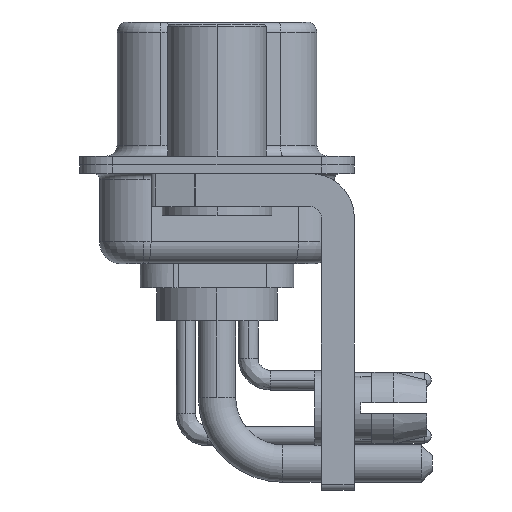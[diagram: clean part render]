
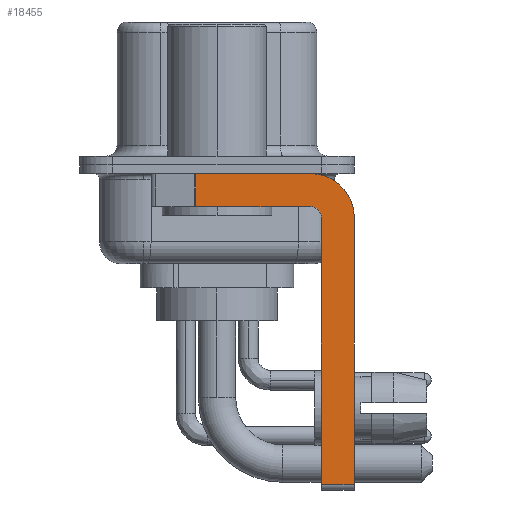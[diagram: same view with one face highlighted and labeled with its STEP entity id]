
A CAD part, left-side view. The second image highlights one B-rep face of the part: STEP entity #18455.
In plain terms, the highlighted planar face has unit normal (-1, 0, 0).
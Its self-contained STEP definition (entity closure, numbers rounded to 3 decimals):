
#10 = VECTOR ( 'NONE', #18727, 1000. ) ;
#968 = VERTEX_POINT ( 'NONE', #21415 ) ;
#1246 = LINE ( 'NONE', #16318, #1496 ) ;
#1315 = ORIENTED_EDGE ( 'NONE', *, *, #11298, .F. ) ;
#1330 = DIRECTION ( 'NONE',  ( 0., 0., -1. ) ) ;
#1350 = DIRECTION ( 'NONE',  ( 0., 0., -1. ) ) ;
#1496 = VECTOR ( 'NONE', #17808, 1000. ) ;
#1505 = LINE ( 'NONE', #12871, #17289 ) ;
#2481 = CARTESIAN_POINT ( 'NONE',  ( -2.9, 0.978, -0.4 ) ) ;
#2623 = CARTESIAN_POINT ( 'NONE',  ( -2.9, -4.25, -14.55 ) ) ;
#2846 = CARTESIAN_POINT ( 'NONE',  ( -2.9, -4.25, -1.9 ) ) ;
#3476 = CARTESIAN_POINT ( 'NONE',  ( -2.9, -4.25, -1.9 ) ) ;
#4120 = DIRECTION ( 'NONE',  ( 1., 0., 0. ) ) ;
#4187 = VERTEX_POINT ( 'NONE', #9725 ) ;
#4868 = AXIS2_PLACEMENT_3D ( 'NONE', #15135, #9073, #11061 ) ;
#4994 = AXIS2_PLACEMENT_3D ( 'NONE', #5964, #4120, #1350 ) ;
#5725 = PLANE ( 'NONE',  #4994 ) ;
#5964 = CARTESIAN_POINT ( 'NONE',  ( -2.9, -4.25, -2.4 ) ) ;
#6555 = DIRECTION ( 'NONE',  ( 0., 1., 0. ) ) ;
#6607 = VERTEX_POINT ( 'NONE', #8759 ) ;
#7018 = LINE ( 'NONE', #11090, #13423 ) ;
#7378 = CARTESIAN_POINT ( 'NONE',  ( -2.9, -6.25, -14.55 ) ) ;
#7439 = EDGE_CURVE ( 'NONE', #19165, #968, #1246, .T. ) ;
#7644 = ORIENTED_EDGE ( 'NONE', *, *, #14174, .F. ) ;
#8012 = DIRECTION ( 'NONE',  ( 0., 0., -1. ) ) ;
#8060 = EDGE_CURVE ( 'NONE', #4187, #6607, #10602, .T. ) ;
#8229 = ORIENTED_EDGE ( 'NONE', *, *, #8060, .F. ) ;
#8239 = VERTEX_POINT ( 'NONE', #7378 ) ;
#8759 = CARTESIAN_POINT ( 'NONE',  ( -2.9, -6.25, -2.4 ) ) ;
#9073 = DIRECTION ( 'NONE',  ( -1., 0., 0. ) ) ;
#9194 = VECTOR ( 'NONE', #15837, 1000. ) ;
#9725 = CARTESIAN_POINT ( 'NONE',  ( -2.9, -4.25, -0.4 ) ) ;
#10111 = DIRECTION ( 'NONE',  ( 1., 0., 0. ) ) ;
#10205 = AXIS2_PLACEMENT_3D ( 'NONE', #19502, #10111, #8012 ) ;
#10602 = CIRCLE ( 'NONE', #10205, 2. ) ;
#11061 = DIRECTION ( 'NONE',  ( 0., 0., 1. ) ) ;
#11090 = CARTESIAN_POINT ( 'NONE',  ( -2.9, 0.978, -1.9 ) ) ;
#11298 = EDGE_CURVE ( 'NONE', #6607, #8239, #18123, .T. ) ;
#12346 = ORIENTED_EDGE ( 'NONE', *, *, #15623, .T. ) ;
#12871 = CARTESIAN_POINT ( 'NONE',  ( -2.9, 3., -0.4 ) ) ;
#13423 = VECTOR ( 'NONE', #1330, 1000. ) ;
#13543 = CIRCLE ( 'NONE', #4868, 0.5 ) ;
#14165 = EDGE_LOOP ( 'NONE', ( #16542, #21817, #15856, #7644, #23378, #12346, #1315, #8229 ) ) ;
#14174 = EDGE_CURVE ( 'NONE', #968, #20871, #13543, .T. ) ;
#15025 = CARTESIAN_POINT ( 'NONE',  ( -2.9, -6.25, -2.4 ) ) ;
#15135 = CARTESIAN_POINT ( 'NONE',  ( -2.9, -4.25, -2.4 ) ) ;
#15345 = FACE_OUTER_BOUND ( 'NONE', #14165, .T. ) ;
#15623 = EDGE_CURVE ( 'NONE', #19165, #8239, #24417, .T. ) ;
#15837 = DIRECTION ( 'NONE',  ( 0., -1., 0. ) ) ;
#15856 = ORIENTED_EDGE ( 'NONE', *, *, #16265, .F. ) ;
#16173 = VERTEX_POINT ( 'NONE', #2481 ) ;
#16265 = EDGE_CURVE ( 'NONE', #20871, #18602, #23497, .T. ) ;
#16318 = CARTESIAN_POINT ( 'NONE',  ( -2.9, -4.75, -14.8 ) ) ;
#16542 = ORIENTED_EDGE ( 'NONE', *, *, #21924, .F. ) ;
#16732 = VECTOR ( 'NONE', #6555, 1000. ) ;
#17289 = VECTOR ( 'NONE', #18198, 1000. ) ;
#17302 = CARTESIAN_POINT ( 'NONE',  ( -2.9, -4.75, -14.55 ) ) ;
#17808 = DIRECTION ( 'NONE',  ( 0., 0., 1. ) ) ;
#18123 = LINE ( 'NONE', #15025, #10 ) ;
#18198 = DIRECTION ( 'NONE',  ( 0., -1., 0. ) ) ;
#18455 = ADVANCED_FACE ( 'NONE', ( #15345 ), #5725, .F. ) ;
#18602 = VERTEX_POINT ( 'NONE', #19061 ) ;
#18727 = DIRECTION ( 'NONE',  ( 0., 0., -1. ) ) ;
#19061 = CARTESIAN_POINT ( 'NONE',  ( -2.9, 0.978, -1.9 ) ) ;
#19165 = VERTEX_POINT ( 'NONE', #17302 ) ;
#19502 = CARTESIAN_POINT ( 'NONE',  ( -2.9, -4.25, -2.4 ) ) ;
#20871 = VERTEX_POINT ( 'NONE', #3476 ) ;
#21415 = CARTESIAN_POINT ( 'NONE',  ( -2.9, -4.75, -2.4 ) ) ;
#21817 = ORIENTED_EDGE ( 'NONE', *, *, #23950, .T. ) ;
#21924 = EDGE_CURVE ( 'NONE', #16173, #4187, #1505, .T. ) ;
#23378 = ORIENTED_EDGE ( 'NONE', *, *, #7439, .F. ) ;
#23497 = LINE ( 'NONE', #2846, #16732 ) ;
#23950 = EDGE_CURVE ( 'NONE', #16173, #18602, #7018, .T. ) ;
#24417 = LINE ( 'NONE', #2623, #9194 ) ;
